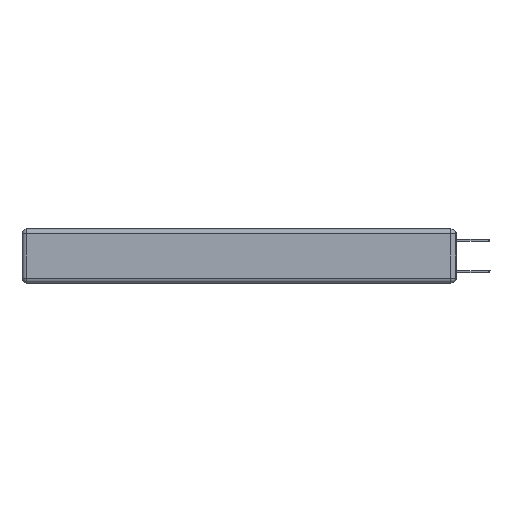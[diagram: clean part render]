
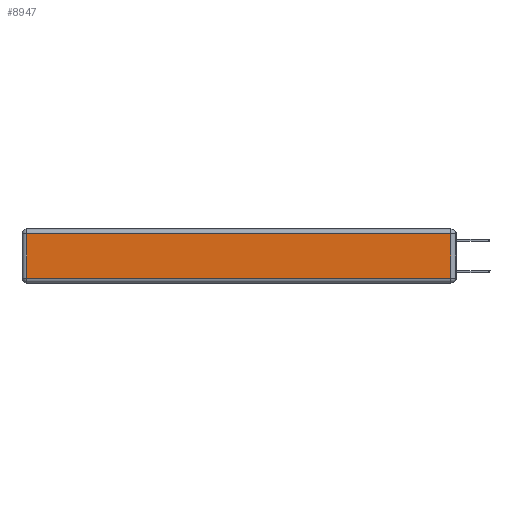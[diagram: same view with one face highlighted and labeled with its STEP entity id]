
A CAD part, left-side view. The second image highlights one B-rep face of the part: STEP entity #8947.
In plain terms, the highlighted planar face has unit normal (-1, 0, 0).
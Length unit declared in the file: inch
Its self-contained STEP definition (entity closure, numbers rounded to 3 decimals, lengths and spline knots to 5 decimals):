
#80 = EDGE_CURVE ( 'NONE', #6485, #3150, #1272, .T. ) ;
#783 = CARTESIAN_POINT ( 'NONE',  ( 0., 0.03, -0.03 ) ) ;
#948 = EDGE_LOOP ( 'NONE', ( #9807, #11354, #2850, #4591 ) ) ;
#1272 = LINE ( 'NONE', #11206, #5183 ) ;
#1994 = DIRECTION ( 'NONE',  ( 0., 1., 0. ) ) ;
#2850 = ORIENTED_EDGE ( 'NONE', *, *, #80, .T. ) ;
#2904 = CARTESIAN_POINT ( 'NONE',  ( 0., 2.72, -0.03 ) ) ;
#2933 = VERTEX_POINT ( 'NONE', #5670 ) ;
#3150 = VERTEX_POINT ( 'NONE', #2904 ) ;
#3166 = AXIS2_PLACEMENT_3D ( 'NONE', #4456, #13678, #6840 ) ;
#3347 = DIRECTION ( 'NONE',  ( 0., 0., 1. ) ) ;
#3777 = DIRECTION ( 'NONE',  ( 0., -1., 0. ) ) ;
#4252 = VERTEX_POINT ( 'NONE', #5564 ) ;
#4429 = CARTESIAN_POINT ( 'NONE',  ( 0., 0.03, -0.343 ) ) ;
#4456 = CARTESIAN_POINT ( 'NONE',  ( 0., 0., -0.343 ) ) ;
#4591 = ORIENTED_EDGE ( 'NONE', *, *, #6330, .T. ) ;
#4762 = CARTESIAN_POINT ( 'NONE',  ( 0., 0., -0.313 ) ) ;
#5183 = VECTOR ( 'NONE', #1994, 39.37008 ) ;
#5309 = VECTOR ( 'NONE', #3347, 39.37008 ) ;
#5491 = LINE ( 'NONE', #4762, #13193 ) ;
#5564 = CARTESIAN_POINT ( 'NONE',  ( 0., 0.03, -0.313 ) ) ;
#5670 = CARTESIAN_POINT ( 'NONE',  ( 0., 2.72, -0.313 ) ) ;
#6330 = EDGE_CURVE ( 'NONE', #3150, #2933, #8750, .T. ) ;
#6485 = VERTEX_POINT ( 'NONE', #783 ) ;
#6840 = DIRECTION ( 'NONE',  ( 0., 0., 1. ) ) ;
#7061 = EDGE_CURVE ( 'NONE', #2933, #4252, #5491, .T. ) ;
#7314 = CARTESIAN_POINT ( 'NONE',  ( 0., 2.72, -0.343 ) ) ;
#8603 = DIRECTION ( 'NONE',  ( 0., 0., -1. ) ) ;
#8750 = LINE ( 'NONE', #7314, #14414 ) ;
#8947 = ADVANCED_FACE ( 'NONE', ( #10478 ), #11369, .T. ) ;
#9807 = ORIENTED_EDGE ( 'NONE', *, *, #7061, .T. ) ;
#10478 = FACE_OUTER_BOUND ( 'NONE', #948, .T. ) ;
#11206 = CARTESIAN_POINT ( 'NONE',  ( 0., 2.75, -0.03 ) ) ;
#11354 = ORIENTED_EDGE ( 'NONE', *, *, #14559, .T. ) ;
#11369 = PLANE ( 'NONE',  #3166 ) ;
#11405 = LINE ( 'NONE', #4429, #5309 ) ;
#13193 = VECTOR ( 'NONE', #3777, 39.37008 ) ;
#13678 = DIRECTION ( 'NONE',  ( -1., 0., 0. ) ) ;
#14414 = VECTOR ( 'NONE', #8603, 39.37008 ) ;
#14559 = EDGE_CURVE ( 'NONE', #4252, #6485, #11405, .T. ) ;
